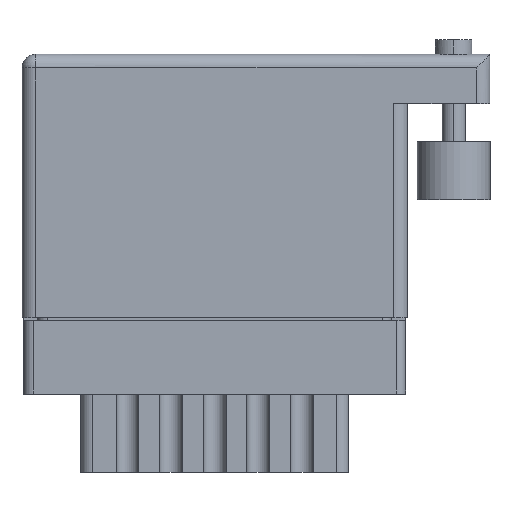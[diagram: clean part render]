
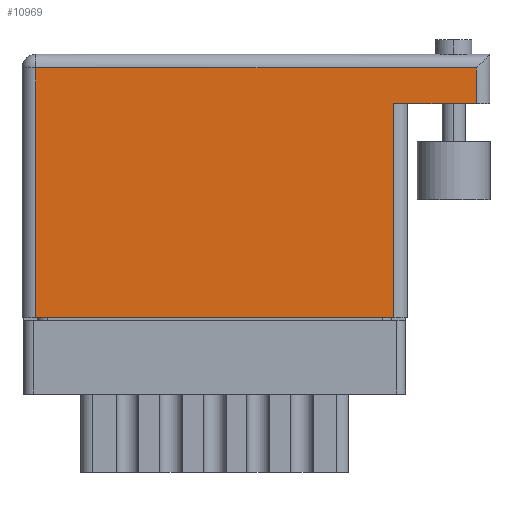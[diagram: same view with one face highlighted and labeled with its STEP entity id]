
A CAD part, front view. The second image highlights one B-rep face of the part: STEP entity #10969.
In plain terms, the highlighted face is planar.
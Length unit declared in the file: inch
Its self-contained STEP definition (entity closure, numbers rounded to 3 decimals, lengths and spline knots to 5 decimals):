
#391 = DIRECTION ( 'NONE',  ( -1., 0., 0. ) ) ;
#734 = CARTESIAN_POINT ( 'NONE',  ( 0.047, 0., 0. ) ) ;
#752 = CARTESIAN_POINT ( 'NONE',  ( 1.562, 0.906, 0. ) ) ;
#811 = VERTEX_POINT ( 'NONE', #24723 ) ;
#838 = CARTESIAN_POINT ( 'NONE',  ( 1.278, 0.736, 0. ) ) ;
#1509 = ORIENTED_EDGE ( 'NONE', *, *, #9027, .T. ) ;
#1632 = VERTEX_POINT ( 'NONE', #21052 ) ;
#2323 = PLANE ( 'NONE',  #27038 ) ;
#2820 = VECTOR ( 'NONE', #21359, 39.37008 ) ;
#3439 = VECTOR ( 'NONE', #11155, 39.37008 ) ;
#3763 = EDGE_CURVE ( 'NONE', #1632, #12084, #26909, .T. ) ;
#4043 = CARTESIAN_POINT ( 'NONE',  ( 0., 0., 0. ) ) ;
#4160 = VECTOR ( 'NONE', #6231, 39.37008 ) ;
#6231 = DIRECTION ( 'NONE',  ( -1., 0., 0. ) ) ;
#7265 = LINE ( 'NONE', #9260, #2820 ) ;
#8082 = ORIENTED_EDGE ( 'NONE', *, *, #3763, .T. ) ;
#9027 = EDGE_CURVE ( 'NONE', #22011, #811, #25098, .T. ) ;
#9260 = CARTESIAN_POINT ( 'NONE',  ( 1.278, 0.736, 0. ) ) ;
#9471 = CARTESIAN_POINT ( 'NONE',  ( 0., 0.906, 0. ) ) ;
#9861 = CARTESIAN_POINT ( 'NONE',  ( 1.562, 0.859, 0. ) ) ;
#10761 = VECTOR ( 'NONE', #391, 39.37008 ) ;
#10969 = ADVANCED_FACE ( 'NONE', ( #23149 ), #2323, .F. ) ;
#11155 = DIRECTION ( 'NONE',  ( 1., 0., 0. ) ) ;
#12084 = VERTEX_POINT ( 'NONE', #9861 ) ;
#12701 = LINE ( 'NONE', #27576, #4160 ) ;
#12824 = VERTEX_POINT ( 'NONE', #838 ) ;
#12962 = EDGE_CURVE ( 'NONE', #13045, #22011, #29341, .T. ) ;
#13045 = VERTEX_POINT ( 'NONE', #22389 ) ;
#13838 = EDGE_LOOP ( 'NONE', ( #1509, #18756, #25547, #8082, #29067, #22407 ) ) ;
#14516 = CARTESIAN_POINT ( 'NONE',  ( 1.609, 0.736, 0. ) ) ;
#15635 = DIRECTION ( 'NONE',  ( 0., -1., 0. ) ) ;
#17049 = EDGE_CURVE ( 'NONE', #1632, #12824, #20334, .T. ) ;
#17075 = VECTOR ( 'NONE', #28861, 39.37008 ) ;
#18424 = DIRECTION ( 'NONE',  ( 0., 0., -1. ) ) ;
#18756 = ORIENTED_EDGE ( 'NONE', *, *, #22037, .T. ) ;
#20334 = LINE ( 'NONE', #14516, #10761 ) ;
#20722 = DIRECTION ( 'NONE',  ( -1., 0., 0. ) ) ;
#21052 = CARTESIAN_POINT ( 'NONE',  ( 1.562, 0.736, 0. ) ) ;
#21359 = DIRECTION ( 'NONE',  ( 0., 1., 0. ) ) ;
#22011 = VERTEX_POINT ( 'NONE', #25331 ) ;
#22037 = EDGE_CURVE ( 'NONE', #811, #12824, #7265, .T. ) ;
#22389 = CARTESIAN_POINT ( 'NONE',  ( 0.047, 0.859, 0. ) ) ;
#22407 = ORIENTED_EDGE ( 'NONE', *, *, #12962, .T. ) ;
#22773 = VECTOR ( 'NONE', #15635, 39.37008 ) ;
#23149 = FACE_OUTER_BOUND ( 'NONE', #13838, .T. ) ;
#24538 = EDGE_CURVE ( 'NONE', #12084, #13045, #12701, .T. ) ;
#24723 = CARTESIAN_POINT ( 'NONE',  ( 1.278, 0., 0. ) ) ;
#25098 = LINE ( 'NONE', #4043, #3439 ) ;
#25331 = CARTESIAN_POINT ( 'NONE',  ( 0.047, 0., 0. ) ) ;
#25547 = ORIENTED_EDGE ( 'NONE', *, *, #17049, .F. ) ;
#26909 = LINE ( 'NONE', #752, #17075 ) ;
#27038 = AXIS2_PLACEMENT_3D ( 'NONE', #9471, #18424, #20722 ) ;
#27576 = CARTESIAN_POINT ( 'NONE',  ( 0., 0.859, 0. ) ) ;
#28861 = DIRECTION ( 'NONE',  ( 0., 1., 0. ) ) ;
#29067 = ORIENTED_EDGE ( 'NONE', *, *, #24538, .T. ) ;
#29341 = LINE ( 'NONE', #734, #22773 ) ;
